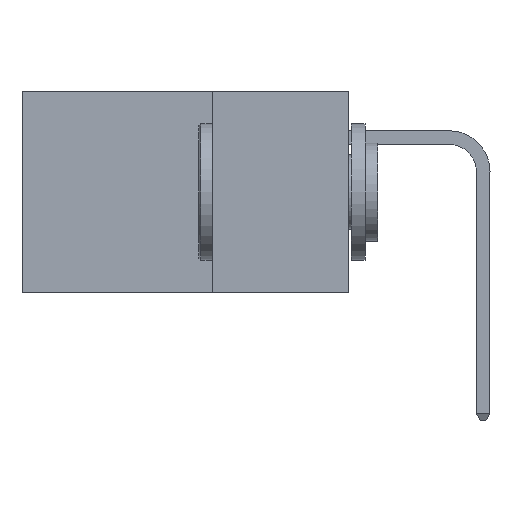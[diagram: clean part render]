
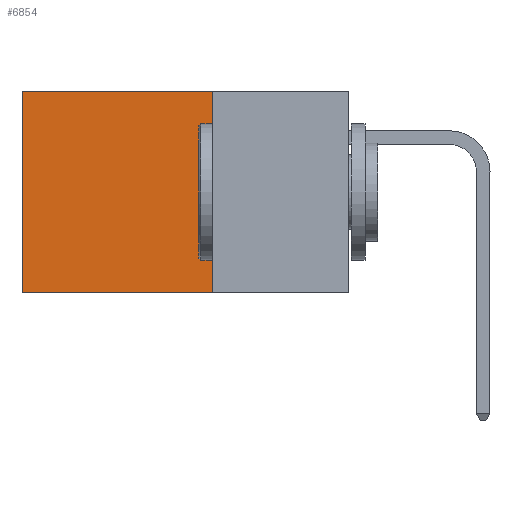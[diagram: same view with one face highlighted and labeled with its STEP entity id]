
A CAD part, left-side view. The second image highlights one B-rep face of the part: STEP entity #6854.
In plain terms, the highlighted planar face has unit normal (-1, 0, 0).
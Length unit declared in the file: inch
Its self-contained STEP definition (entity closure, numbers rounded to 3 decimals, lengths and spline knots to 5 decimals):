
#774 = VERTEX_POINT ( 'NONE', #5555 ) ;
#939 = ORIENTED_EDGE ( 'NONE', *, *, #2990, .F. ) ;
#1012 = CARTESIAN_POINT ( 'NONE',  ( 0.2875, 0.25, -0.37 ) ) ;
#1108 = FACE_OUTER_BOUND ( 'NONE', #4373, .T. ) ;
#1542 = DIRECTION ( 'NONE',  ( 0., 1., 0. ) ) ;
#1712 = CARTESIAN_POINT ( 'NONE',  ( 0.2875, 0.25, -0.37 ) ) ;
#2181 = EDGE_CURVE ( 'NONE', #12340, #5242, #11292, .T. ) ;
#2292 = PLANE ( 'NONE',  #2306 ) ;
#2306 = AXIS2_PLACEMENT_3D ( 'NONE', #9607, #13040, #10528 ) ;
#2990 = EDGE_CURVE ( 'NONE', #5242, #774, #6807, .T. ) ;
#3338 = ORIENTED_EDGE ( 'NONE', *, *, #12240, .T. ) ;
#3615 = ORIENTED_EDGE ( 'NONE', *, *, #7972, .T. ) ;
#4291 = CARTESIAN_POINT ( 'NONE',  ( 0.2875, 0.6, 0. ) ) ;
#4373 = EDGE_LOOP ( 'NONE', ( #3338, #939, #4993, #3615 ) ) ;
#4484 = DIRECTION ( 'NONE',  ( 0., 1., 0. ) ) ;
#4993 = ORIENTED_EDGE ( 'NONE', *, *, #2181, .F. ) ;
#5146 = LINE ( 'NONE', #11271, #8126 ) ;
#5242 = VERTEX_POINT ( 'NONE', #1012 ) ;
#5555 = CARTESIAN_POINT ( 'NONE',  ( 0.2875, 0.6, -0.37 ) ) ;
#5872 = VECTOR ( 'NONE', #7127, 39.37008 ) ;
#6307 = VECTOR ( 'NONE', #11108, 39.37008 ) ;
#6460 = CARTESIAN_POINT ( 'NONE',  ( 0.2875, 0.25, 0. ) ) ;
#6807 = LINE ( 'NONE', #1712, #9150 ) ;
#6854 = ADVANCED_FACE ( 'NONE', ( #1108 ), #2292, .F. ) ;
#7127 = DIRECTION ( 'NONE',  ( 0., 0., -1. ) ) ;
#7219 = CARTESIAN_POINT ( 'NONE',  ( 0.2875, 0.25, 0. ) ) ;
#7972 = EDGE_CURVE ( 'NONE', #12340, #10177, #5146, .T. ) ;
#8126 = VECTOR ( 'NONE', #4484, 39.37008 ) ;
#8661 = LINE ( 'NONE', #4291, #6307 ) ;
#9150 = VECTOR ( 'NONE', #1542, 39.37008 ) ;
#9607 = CARTESIAN_POINT ( 'NONE',  ( 0.2875, 0.25, 0. ) ) ;
#10177 = VERTEX_POINT ( 'NONE', #12495 ) ;
#10528 = DIRECTION ( 'NONE',  ( 0., 0., -1. ) ) ;
#11108 = DIRECTION ( 'NONE',  ( 0., 0., -1. ) ) ;
#11271 = CARTESIAN_POINT ( 'NONE',  ( 0.2875, 0.25, 0. ) ) ;
#11292 = LINE ( 'NONE', #7219, #5872 ) ;
#12240 = EDGE_CURVE ( 'NONE', #10177, #774, #8661, .T. ) ;
#12340 = VERTEX_POINT ( 'NONE', #6460 ) ;
#12495 = CARTESIAN_POINT ( 'NONE',  ( 0.2875, 0.6, 0. ) ) ;
#13040 = DIRECTION ( 'NONE',  ( 1., 0., 0. ) ) ;
